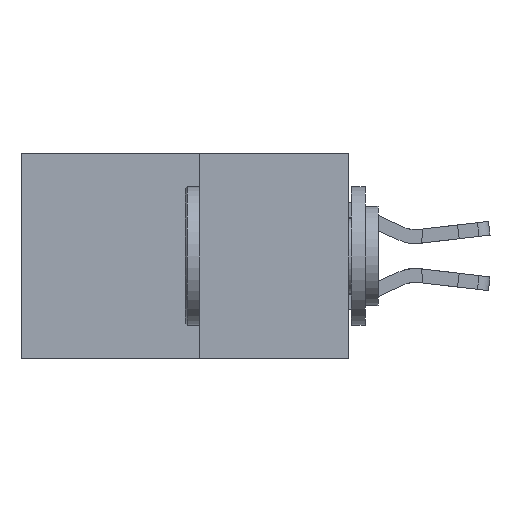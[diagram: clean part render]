
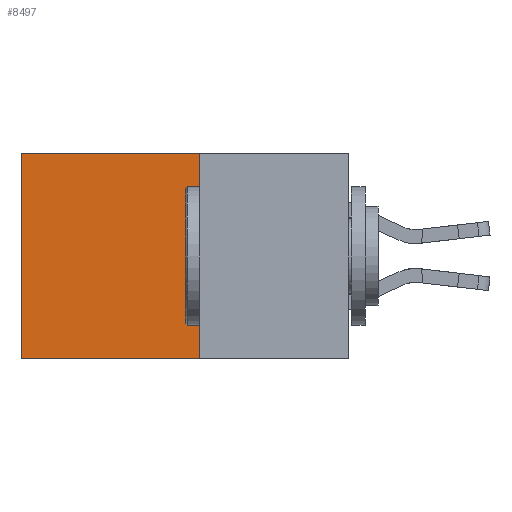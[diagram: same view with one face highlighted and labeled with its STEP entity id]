
A CAD part, left-side view. The second image highlights one B-rep face of the part: STEP entity #8497.
In plain terms, the highlighted planar face has unit normal (-1, 0, 0).
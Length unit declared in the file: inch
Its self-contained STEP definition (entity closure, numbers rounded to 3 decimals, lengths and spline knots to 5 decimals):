
#982 = EDGE_CURVE ( 'NONE', #6036, #26858, #7367, .T. ) ;
#1572 = EDGE_CURVE ( 'NONE', #6036, #19020, #4895, .T. ) ;
#2046 = ORIENTED_EDGE ( 'NONE', *, *, #1572, .T. ) ;
#2294 = CARTESIAN_POINT ( 'NONE',  ( 0.277, 0.27, 0. ) ) ;
#3187 = CARTESIAN_POINT ( 'NONE',  ( 0.277, 0.27, 0. ) ) ;
#3588 = PLANE ( 'NONE',  #25949 ) ;
#4350 = DIRECTION ( 'NONE',  ( 0., 0., -1. ) ) ;
#4881 = VERTEX_POINT ( 'NONE', #26046 ) ;
#4895 = LINE ( 'NONE', #2294, #11609 ) ;
#4971 = VECTOR ( 'NONE', #24632, 39.37008 ) ;
#5120 = LINE ( 'NONE', #25074, #10438 ) ;
#6036 = VERTEX_POINT ( 'NONE', #3187 ) ;
#7367 = LINE ( 'NONE', #16627, #24492 ) ;
#8080 = ORIENTED_EDGE ( 'NONE', *, *, #982, .F. ) ;
#8169 = DIRECTION ( 'NONE',  ( 1., 0., 0. ) ) ;
#8497 = ADVANCED_FACE ( 'NONE', ( #10781 ), #3588, .F. ) ;
#8592 = EDGE_LOOP ( 'NONE', ( #9931, #23671, #8080, #2046 ) ) ;
#9931 = ORIENTED_EDGE ( 'NONE', *, *, #17067, .T. ) ;
#10438 = VECTOR ( 'NONE', #13962, 39.37008 ) ;
#10781 = FACE_OUTER_BOUND ( 'NONE', #8592, .T. ) ;
#11299 = CARTESIAN_POINT ( 'NONE',  ( 0.277, 0.59, -0.37 ) ) ;
#11609 = VECTOR ( 'NONE', #20801, 39.37008 ) ;
#11905 = CARTESIAN_POINT ( 'NONE',  ( 0.277, 0.59, 0. ) ) ;
#13962 = DIRECTION ( 'NONE',  ( 0., 1., 0. ) ) ;
#13999 = EDGE_CURVE ( 'NONE', #26858, #4881, #5120, .T. ) ;
#16519 = CARTESIAN_POINT ( 'NONE',  ( 0.277, 0.27, -0.37 ) ) ;
#16627 = CARTESIAN_POINT ( 'NONE',  ( 0.277, 0.27, -0.37 ) ) ;
#16914 = LINE ( 'NONE', #11299, #4971 ) ;
#17067 = EDGE_CURVE ( 'NONE', #19020, #4881, #16914, .T. ) ;
#19020 = VERTEX_POINT ( 'NONE', #11905 ) ;
#20801 = DIRECTION ( 'NONE',  ( 0., 1., 0. ) ) ;
#21564 = CARTESIAN_POINT ( 'NONE',  ( 0.277, 0.27, -0.37 ) ) ;
#23671 = ORIENTED_EDGE ( 'NONE', *, *, #13999, .F. ) ;
#23796 = DIRECTION ( 'NONE',  ( 0., 0., -1. ) ) ;
#24492 = VECTOR ( 'NONE', #4350, 39.37008 ) ;
#24632 = DIRECTION ( 'NONE',  ( 0., 0., -1. ) ) ;
#25074 = CARTESIAN_POINT ( 'NONE',  ( 0.277, 0.27, -0.37 ) ) ;
#25949 = AXIS2_PLACEMENT_3D ( 'NONE', #21564, #8169, #23796 ) ;
#26046 = CARTESIAN_POINT ( 'NONE',  ( 0.277, 0.59, -0.37 ) ) ;
#26858 = VERTEX_POINT ( 'NONE', #16519 ) ;
